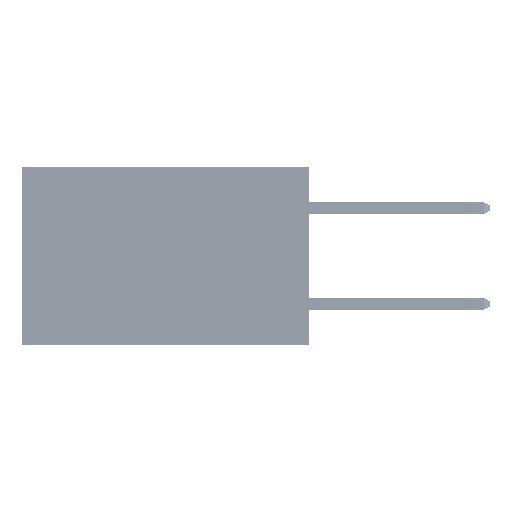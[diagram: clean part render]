
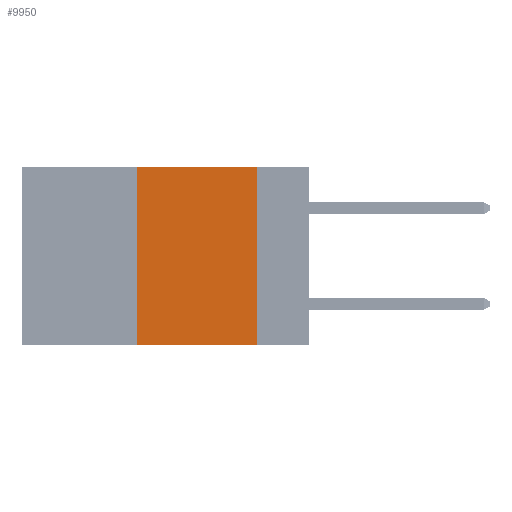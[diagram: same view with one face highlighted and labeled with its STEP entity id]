
A CAD part, left-side view. The second image highlights one B-rep face of the part: STEP entity #9950.
In plain terms, the highlighted planar face has unit normal (-1, 0, 0).
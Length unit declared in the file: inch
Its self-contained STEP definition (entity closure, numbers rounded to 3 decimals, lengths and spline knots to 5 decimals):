
#234 = ORIENTED_EDGE ( 'NONE', *, *, #39039, .F. ) ;
#1516 = ORIENTED_EDGE ( 'NONE', *, *, #38732, .T. ) ;
#3564 = LINE ( 'NONE', #45044, #12793 ) ;
#4689 = LINE ( 'NONE', #40677, #13889 ) ;
#5883 = LINE ( 'NONE', #12939, #46109 ) ;
#6691 = EDGE_CURVE ( 'NONE', #35919, #10936, #4689, .T. ) ;
#7151 = VERTEX_POINT ( 'NONE', #43358 ) ;
#9950 = ADVANCED_FACE ( 'NONE', ( #41632 ), #17785, .F. ) ;
#10936 = VERTEX_POINT ( 'NONE', #46400 ) ;
#11670 = CARTESIAN_POINT ( 'NONE',  ( 0., 0.36, 0. ) ) ;
#12010 = VECTOR ( 'NONE', #25103, 39.37008 ) ;
#12793 = VECTOR ( 'NONE', #25658, 39.37008 ) ;
#12939 = CARTESIAN_POINT ( 'NONE',  ( 0., 0.6, -0.37 ) ) ;
#13889 = VECTOR ( 'NONE', #21304, 39.37008 ) ;
#17785 = PLANE ( 'NONE',  #39577 ) ;
#21304 = DIRECTION ( 'NONE',  ( 0., -1., 0. ) ) ;
#25103 = DIRECTION ( 'NONE',  ( 0., 0., 1. ) ) ;
#25576 = DIRECTION ( 'NONE',  ( 0., 0., -1. ) ) ;
#25658 = DIRECTION ( 'NONE',  ( 0., 0., -1. ) ) ;
#27226 = ORIENTED_EDGE ( 'NONE', *, *, #46055, .F. ) ;
#27800 = EDGE_LOOP ( 'NONE', ( #27226, #41238, #234, #1516 ) ) ;
#31091 = DIRECTION ( 'NONE',  ( 0., -1., 0. ) ) ;
#32714 = LINE ( 'NONE', #44490, #12010 ) ;
#35374 = VERTEX_POINT ( 'NONE', #48447 ) ;
#35919 = VERTEX_POINT ( 'NONE', #11670 ) ;
#38732 = EDGE_CURVE ( 'NONE', #35374, #7151, #5883, .T. ) ;
#39039 = EDGE_CURVE ( 'NONE', #35374, #35919, #32714, .T. ) ;
#39577 = AXIS2_PLACEMENT_3D ( 'NONE', #44964, #48826, #25576 ) ;
#40677 = CARTESIAN_POINT ( 'NONE',  ( 0., 0.6, 0. ) ) ;
#41238 = ORIENTED_EDGE ( 'NONE', *, *, #6691, .F. ) ;
#41632 = FACE_OUTER_BOUND ( 'NONE', #27800, .T. ) ;
#43358 = CARTESIAN_POINT ( 'NONE',  ( 0., 0.11, -0.37 ) ) ;
#44490 = CARTESIAN_POINT ( 'NONE',  ( 0., 0.36, 0. ) ) ;
#44964 = CARTESIAN_POINT ( 'NONE',  ( 0., 0.6, 0. ) ) ;
#45044 = CARTESIAN_POINT ( 'NONE',  ( 0., 0.11, 0. ) ) ;
#46055 = EDGE_CURVE ( 'NONE', #10936, #7151, #3564, .T. ) ;
#46109 = VECTOR ( 'NONE', #31091, 39.37008 ) ;
#46400 = CARTESIAN_POINT ( 'NONE',  ( 0., 0.11, 0. ) ) ;
#48447 = CARTESIAN_POINT ( 'NONE',  ( 0., 0.36, -0.37 ) ) ;
#48826 = DIRECTION ( 'NONE',  ( 1., 0., 0. ) ) ;
